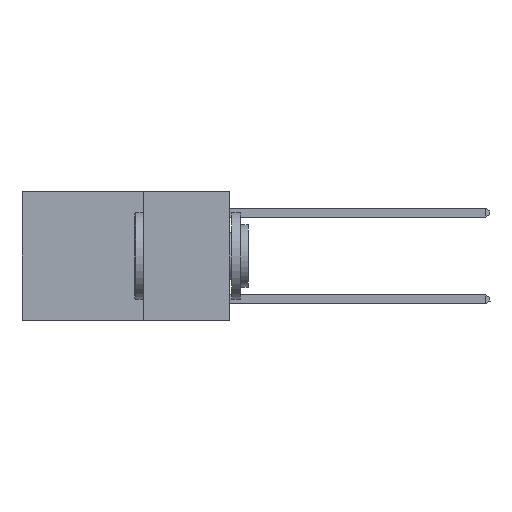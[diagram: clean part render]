
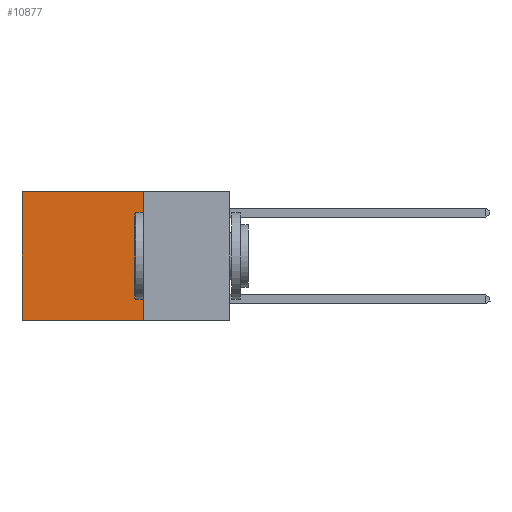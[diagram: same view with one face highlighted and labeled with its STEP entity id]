
A CAD part, left-side view. The second image highlights one B-rep face of the part: STEP entity #10877.
In plain terms, the highlighted planar face has unit normal (-1, 0, 0).
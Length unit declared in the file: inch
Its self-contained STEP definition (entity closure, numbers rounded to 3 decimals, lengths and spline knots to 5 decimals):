
#426 = CARTESIAN_POINT ( 'NONE',  ( 0.2625, 0.25, -0.37 ) ) ;
#481 = ORIENTED_EDGE ( 'NONE', *, *, #6167, .F. ) ;
#655 = VERTEX_POINT ( 'NONE', #1418 ) ;
#871 = LINE ( 'NONE', #426, #7001 ) ;
#931 = EDGE_CURVE ( 'NONE', #6683, #6303, #871, .T. ) ;
#1168 = CARTESIAN_POINT ( 'NONE',  ( 0.2625, 0.25, 0. ) ) ;
#1216 = VECTOR ( 'NONE', #9468, 39.37008 ) ;
#1418 = CARTESIAN_POINT ( 'NONE',  ( 0.2625, 0.6, 0. ) ) ;
#1615 = CARTESIAN_POINT ( 'NONE',  ( 0.2625, 0.25, 0. ) ) ;
#1655 = VERTEX_POINT ( 'NONE', #7753 ) ;
#2794 = EDGE_LOOP ( 'NONE', ( #4119, #3270, #481, #9335 ) ) ;
#3270 = ORIENTED_EDGE ( 'NONE', *, *, #931, .F. ) ;
#3373 = CARTESIAN_POINT ( 'NONE',  ( 0.2625, 0.25, -0.37 ) ) ;
#3865 = DIRECTION ( 'NONE',  ( 0., 1., 0. ) ) ;
#4119 = ORIENTED_EDGE ( 'NONE', *, *, #8274, .T. ) ;
#4837 = CARTESIAN_POINT ( 'NONE',  ( 0.2625, 0.25, 0. ) ) ;
#4928 = LINE ( 'NONE', #1615, #7644 ) ;
#5975 = DIRECTION ( 'NONE',  ( 0., 0., -1. ) ) ;
#6167 = EDGE_CURVE ( 'NONE', #1655, #6683, #14486, .T. ) ;
#6303 = VERTEX_POINT ( 'NONE', #9527 ) ;
#6683 = VERTEX_POINT ( 'NONE', #3373 ) ;
#6916 = FACE_OUTER_BOUND ( 'NONE', #2794, .T. ) ;
#7001 = VECTOR ( 'NONE', #12374, 39.37008 ) ;
#7644 = VECTOR ( 'NONE', #3865, 39.37008 ) ;
#7753 = CARTESIAN_POINT ( 'NONE',  ( 0.2625, 0.25, 0. ) ) ;
#8080 = DIRECTION ( 'NONE',  ( 0., 0., -1. ) ) ;
#8274 = EDGE_CURVE ( 'NONE', #655, #6303, #13260, .T. ) ;
#9335 = ORIENTED_EDGE ( 'NONE', *, *, #11599, .T. ) ;
#9468 = DIRECTION ( 'NONE',  ( 0., 0., -1. ) ) ;
#9527 = CARTESIAN_POINT ( 'NONE',  ( 0.2625, 0.6, -0.37 ) ) ;
#10877 = ADVANCED_FACE ( 'NONE', ( #6916 ), #11652, .F. ) ;
#11599 = EDGE_CURVE ( 'NONE', #1655, #655, #4928, .T. ) ;
#11652 = PLANE ( 'NONE',  #14275 ) ;
#12374 = DIRECTION ( 'NONE',  ( 0., 1., 0. ) ) ;
#12727 = DIRECTION ( 'NONE',  ( 1., 0., 0. ) ) ;
#13260 = LINE ( 'NONE', #13825, #1216 ) ;
#13815 = VECTOR ( 'NONE', #8080, 39.37008 ) ;
#13825 = CARTESIAN_POINT ( 'NONE',  ( 0.2625, 0.6, 0. ) ) ;
#14275 = AXIS2_PLACEMENT_3D ( 'NONE', #4837, #12727, #5975 ) ;
#14486 = LINE ( 'NONE', #1168, #13815 ) ;
